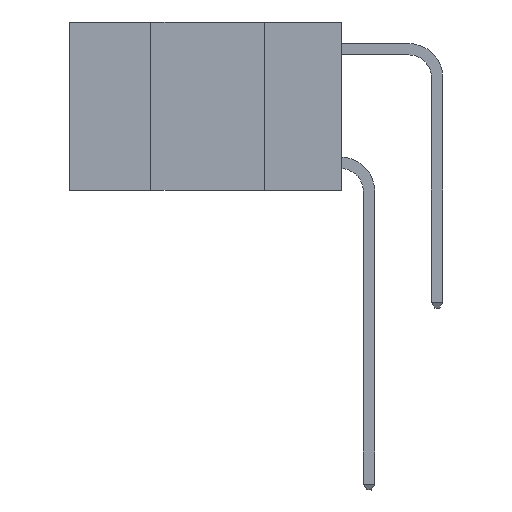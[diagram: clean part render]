
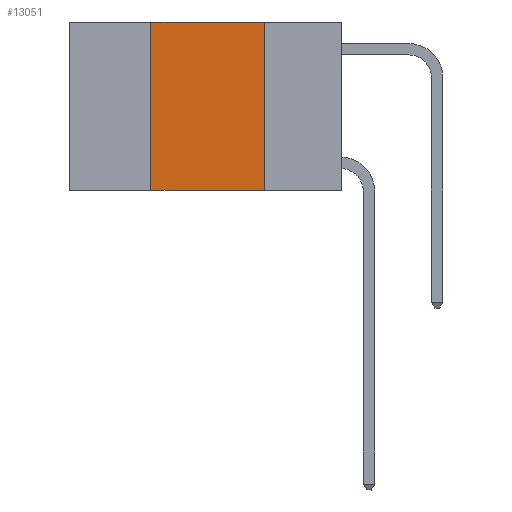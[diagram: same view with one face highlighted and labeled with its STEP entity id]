
A CAD part, left-side view. The second image highlights one B-rep face of the part: STEP entity #13051.
In plain terms, the highlighted planar face has unit normal (-1, 0, 0).
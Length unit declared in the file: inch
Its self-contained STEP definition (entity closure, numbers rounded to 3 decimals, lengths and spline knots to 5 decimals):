
#36 = ORIENTED_EDGE ( 'NONE', *, *, #11135, .T. ) ;
#182 = ORIENTED_EDGE ( 'NONE', *, *, #12039, .F. ) ;
#410 = LINE ( 'NONE', #597, #8860 ) ;
#415 = ORIENTED_EDGE ( 'NONE', *, *, #1895, .F. ) ;
#597 = CARTESIAN_POINT ( 'NONE',  ( 0., 0.42, 0. ) ) ;
#753 = PLANE ( 'NONE',  #5936 ) ;
#1386 = EDGE_CURVE ( 'NONE', #10743, #6402, #410, .T. ) ;
#1478 = VERTEX_POINT ( 'NONE', #7396 ) ;
#1512 = ORIENTED_EDGE ( 'NONE', *, *, #1386, .F. ) ;
#1895 = EDGE_CURVE ( 'NONE', #1478, #13375, #8701, .T. ) ;
#2241 = CARTESIAN_POINT ( 'NONE',  ( 0., 0.42, 0. ) ) ;
#2454 = CARTESIAN_POINT ( 'NONE',  ( 0., 0.17, -0.37 ) ) ;
#2897 = DIRECTION ( 'NONE',  ( 0., 0., 1. ) ) ;
#3980 = VECTOR ( 'NONE', #10969, 39.37008 ) ;
#4329 = LINE ( 'NONE', #9929, #3980 ) ;
#4791 = DIRECTION ( 'NONE',  ( 0., 0., -1. ) ) ;
#5858 = VECTOR ( 'NONE', #4791, 39.37008 ) ;
#5936 = AXIS2_PLACEMENT_3D ( 'NONE', #10560, #12642, #6373 ) ;
#6251 = DIRECTION ( 'NONE',  ( 0., -1., 0. ) ) ;
#6373 = DIRECTION ( 'NONE',  ( 0., 0., -1. ) ) ;
#6402 = VERTEX_POINT ( 'NONE', #2241 ) ;
#7396 = CARTESIAN_POINT ( 'NONE',  ( 0., 0.17, 0. ) ) ;
#8701 = LINE ( 'NONE', #11123, #5858 ) ;
#8791 = CARTESIAN_POINT ( 'NONE',  ( 0., 0.42, -0.37 ) ) ;
#8860 = VECTOR ( 'NONE', #2897, 39.37008 ) ;
#9929 = CARTESIAN_POINT ( 'NONE',  ( 0., 0.6, 0. ) ) ;
#10560 = CARTESIAN_POINT ( 'NONE',  ( 0., 0.6, 0. ) ) ;
#10668 = LINE ( 'NONE', #12524, #13103 ) ;
#10743 = VERTEX_POINT ( 'NONE', #8791 ) ;
#10969 = DIRECTION ( 'NONE',  ( 0., -1., 0. ) ) ;
#11123 = CARTESIAN_POINT ( 'NONE',  ( 0., 0.17, 0. ) ) ;
#11135 = EDGE_CURVE ( 'NONE', #10743, #13375, #10668, .T. ) ;
#12039 = EDGE_CURVE ( 'NONE', #6402, #1478, #4329, .T. ) ;
#12524 = CARTESIAN_POINT ( 'NONE',  ( 0., 0.6, -0.37 ) ) ;
#12642 = DIRECTION ( 'NONE',  ( 1., 0., 0. ) ) ;
#13051 = ADVANCED_FACE ( 'NONE', ( #13203 ), #753, .F. ) ;
#13103 = VECTOR ( 'NONE', #6251, 39.37008 ) ;
#13203 = FACE_OUTER_BOUND ( 'NONE', #13268, .T. ) ;
#13268 = EDGE_LOOP ( 'NONE', ( #415, #182, #1512, #36 ) ) ;
#13375 = VERTEX_POINT ( 'NONE', #2454 ) ;
